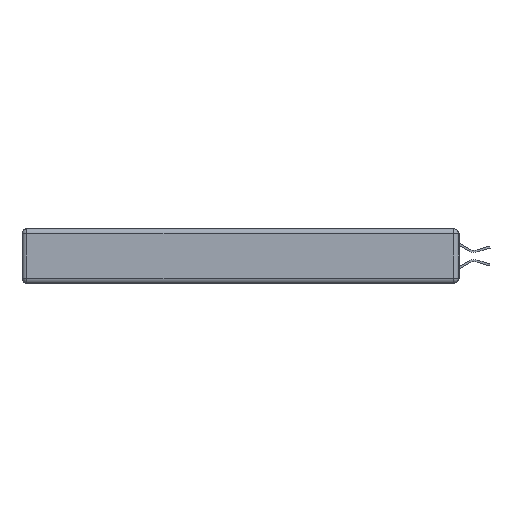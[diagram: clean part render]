
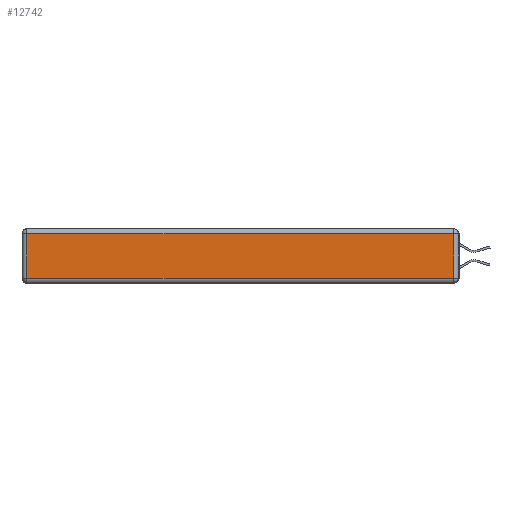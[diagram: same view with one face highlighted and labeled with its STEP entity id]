
A CAD part, left-side view. The second image highlights one B-rep face of the part: STEP entity #12742.
In plain terms, the highlighted planar face has unit normal (-1, 0, 0).
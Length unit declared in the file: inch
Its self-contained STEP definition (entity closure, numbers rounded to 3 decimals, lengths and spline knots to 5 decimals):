
#248 = EDGE_CURVE ( 'NONE', #15956, #16632, #3835, .T. ) ;
#517 = ORIENTED_EDGE ( 'NONE', *, *, #15672, .T. ) ;
#1426 = LINE ( 'NONE', #9113, #3586 ) ;
#1587 = VECTOR ( 'NONE', #7862, 39.37008 ) ;
#1766 = VERTEX_POINT ( 'NONE', #16054 ) ;
#3051 = VERTEX_POINT ( 'NONE', #5207 ) ;
#3456 = DIRECTION ( 'NONE',  ( 0., -1., 0. ) ) ;
#3586 = VECTOR ( 'NONE', #3456, 39.37008 ) ;
#3835 = LINE ( 'NONE', #9741, #1587 ) ;
#5207 = CARTESIAN_POINT ( 'NONE',  ( 0., 0.03, -0.313 ) ) ;
#6405 = EDGE_LOOP ( 'NONE', ( #517, #8856, #9430, #10007 ) ) ;
#7278 = EDGE_CURVE ( 'NONE', #3051, #1766, #23155, .T. ) ;
#7322 = FACE_OUTER_BOUND ( 'NONE', #6405, .T. ) ;
#7862 = DIRECTION ( 'NONE',  ( 0., 0., -1. ) ) ;
#8856 = ORIENTED_EDGE ( 'NONE', *, *, #7278, .T. ) ;
#9113 = CARTESIAN_POINT ( 'NONE',  ( 0., 0., -0.313 ) ) ;
#9430 = ORIENTED_EDGE ( 'NONE', *, *, #24102, .T. ) ;
#9741 = CARTESIAN_POINT ( 'NONE',  ( 0., 2.72, -0.343 ) ) ;
#10007 = ORIENTED_EDGE ( 'NONE', *, *, #248, .T. ) ;
#11451 = CARTESIAN_POINT ( 'NONE',  ( 0., 2.72, -0.03 ) ) ;
#11561 = LINE ( 'NONE', #21146, #15235 ) ;
#12742 = ADVANCED_FACE ( 'NONE', ( #7322 ), #13484, .T. ) ;
#13333 = DIRECTION ( 'NONE',  ( 0., 0., 1. ) ) ;
#13484 = PLANE ( 'NONE',  #21180 ) ;
#14537 = CARTESIAN_POINT ( 'NONE',  ( 0., 2.72, -0.313 ) ) ;
#15024 = DIRECTION ( 'NONE',  ( -1., 0., 0. ) ) ;
#15235 = VECTOR ( 'NONE', #19250, 39.37008 ) ;
#15276 = DIRECTION ( 'NONE',  ( 0., 0., 1. ) ) ;
#15672 = EDGE_CURVE ( 'NONE', #16632, #3051, #1426, .T. ) ;
#15956 = VERTEX_POINT ( 'NONE', #11451 ) ;
#16054 = CARTESIAN_POINT ( 'NONE',  ( 0., 0.03, -0.03 ) ) ;
#16632 = VERTEX_POINT ( 'NONE', #14537 ) ;
#17264 = CARTESIAN_POINT ( 'NONE',  ( 0., 0., -0.343 ) ) ;
#19250 = DIRECTION ( 'NONE',  ( 0., 1., 0. ) ) ;
#21146 = CARTESIAN_POINT ( 'NONE',  ( 0., 2.75, -0.03 ) ) ;
#21180 = AXIS2_PLACEMENT_3D ( 'NONE', #17264, #15024, #15276 ) ;
#21278 = CARTESIAN_POINT ( 'NONE',  ( 0., 0.03, -0.343 ) ) ;
#21768 = VECTOR ( 'NONE', #13333, 39.37008 ) ;
#23155 = LINE ( 'NONE', #21278, #21768 ) ;
#24102 = EDGE_CURVE ( 'NONE', #1766, #15956, #11561, .T. ) ;
